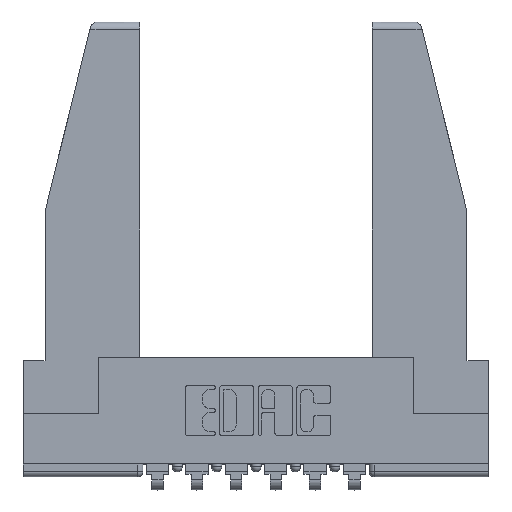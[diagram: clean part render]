
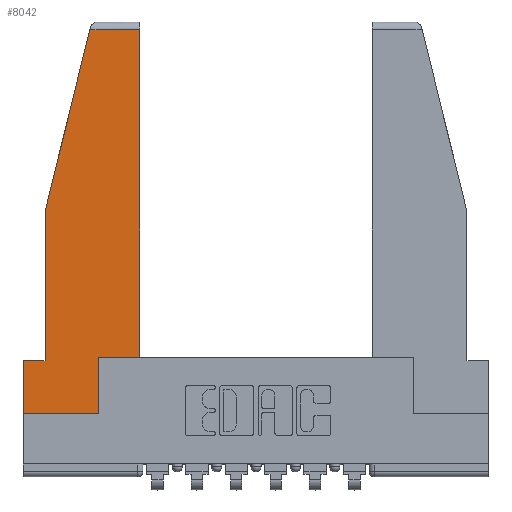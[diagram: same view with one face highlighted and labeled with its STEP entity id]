
A CAD part, top view. The second image highlights one B-rep face of the part: STEP entity #8042.
In plain terms, the highlighted planar face has unit normal (0, 0, 1).
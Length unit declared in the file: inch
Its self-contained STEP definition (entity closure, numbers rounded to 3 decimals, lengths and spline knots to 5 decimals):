
#149 = DIRECTION ( 'NONE',  ( 0., 1., 0. ) ) ;
#506 = EDGE_CURVE ( 'NONE', #4502, #9642, #3231, .T. ) ;
#559 = DIRECTION ( 'NONE',  ( -0.239, -0.971, 0. ) ) ;
#589 = VERTEX_POINT ( 'NONE', #7396 ) ;
#690 = CARTESIAN_POINT ( 'NONE',  ( 0.086, 0.8, 0. ) ) ;
#927 = CARTESIAN_POINT ( 'NONE',  ( 0.2636, 1.52, 0. ) ) ;
#933 = VECTOR ( 'NONE', #2830, 39.37008 ) ;
#1018 = CARTESIAN_POINT ( 'NONE',  ( 0.086, 0.21, 0. ) ) ;
#1309 = LINE ( 'NONE', #6070, #3878 ) ;
#1405 = EDGE_CURVE ( 'NONE', #5147, #3144, #2658, .T. ) ;
#1675 = FACE_OUTER_BOUND ( 'NONE', #10963, .T. ) ;
#1799 = CARTESIAN_POINT ( 'NONE',  ( 0., 0.21, 0. ) ) ;
#1808 = DIRECTION ( 'NONE',  ( 0., 0., 1. ) ) ;
#2299 = VECTOR ( 'NONE', #8438, 39.37008 ) ;
#2321 = DIRECTION ( 'NONE',  ( 1., 0., 0. ) ) ;
#2417 = CARTESIAN_POINT ( 'NONE',  ( 0.461, 0.223, 0. ) ) ;
#2658 = LINE ( 'NONE', #4690, #3226 ) ;
#2830 = DIRECTION ( 'NONE',  ( -1., 0., 0. ) ) ;
#2982 = ORIENTED_EDGE ( 'NONE', *, *, #9877, .T. ) ;
#3100 = VECTOR ( 'NONE', #149, 39.37008 ) ;
#3144 = VERTEX_POINT ( 'NONE', #12222 ) ;
#3226 = VECTOR ( 'NONE', #559, 39.37008 ) ;
#3231 = LINE ( 'NONE', #4208, #3100 ) ;
#3272 = EDGE_CURVE ( 'NONE', #589, #4502, #5633, .T. ) ;
#3565 = CARTESIAN_POINT ( 'NONE',  ( 0.297, 0., 0. ) ) ;
#3636 = PLANE ( 'NONE',  #4230 ) ;
#3766 = DIRECTION ( 'NONE',  ( 1., 0., 0. ) ) ;
#3878 = VECTOR ( 'NONE', #4056, 39.37008 ) ;
#4056 = DIRECTION ( 'NONE',  ( -1., 0., 0. ) ) ;
#4208 = CARTESIAN_POINT ( 'NONE',  ( 0.297, 0., 0. ) ) ;
#4230 = AXIS2_PLACEMENT_3D ( 'NONE', #12423, #1808, #3766 ) ;
#4235 = VERTEX_POINT ( 'NONE', #1018 ) ;
#4462 = EDGE_CURVE ( 'NONE', #9642, #12052, #11236, .T. ) ;
#4502 = VERTEX_POINT ( 'NONE', #3565 ) ;
#4690 = CARTESIAN_POINT ( 'NONE',  ( 0.271, 1.55, 0. ) ) ;
#4838 = ORIENTED_EDGE ( 'NONE', *, *, #4462, .T. ) ;
#5147 = VERTEX_POINT ( 'NONE', #927 ) ;
#5232 = VERTEX_POINT ( 'NONE', #11015 ) ;
#5301 = VECTOR ( 'NONE', #8489, 39.37008 ) ;
#5364 = CARTESIAN_POINT ( 'NONE',  ( 0.461, 0.223, 0. ) ) ;
#5633 = LINE ( 'NONE', #11498, #8528 ) ;
#5769 = EDGE_CURVE ( 'NONE', #3144, #4235, #9608, .T. ) ;
#6070 = CARTESIAN_POINT ( 'NONE',  ( 0., 1.52, 0. ) ) ;
#6345 = LINE ( 'NONE', #5364, #9210 ) ;
#7111 = ORIENTED_EDGE ( 'NONE', *, *, #8446, .T. ) ;
#7396 = CARTESIAN_POINT ( 'NONE',  ( 0., 0., 0. ) ) ;
#7596 = DIRECTION ( 'NONE',  ( 1., 0., 0. ) ) ;
#7936 = ORIENTED_EDGE ( 'NONE', *, *, #3272, .T. ) ;
#8042 = ADVANCED_FACE ( 'NONE', ( #1675 ), #3636, .T. ) ;
#8073 = VERTEX_POINT ( 'NONE', #9675 ) ;
#8438 = DIRECTION ( 'NONE',  ( 0., -1., 0. ) ) ;
#8446 = EDGE_CURVE ( 'NONE', #12052, #5232, #6345, .T. ) ;
#8489 = DIRECTION ( 'NONE',  ( 0., -1., 0. ) ) ;
#8528 = VECTOR ( 'NONE', #7596, 39.37008 ) ;
#9210 = VECTOR ( 'NONE', #9329, 39.37008 ) ;
#9329 = DIRECTION ( 'NONE',  ( 0., 1., 0. ) ) ;
#9608 = LINE ( 'NONE', #690, #2299 ) ;
#9642 = VERTEX_POINT ( 'NONE', #11294 ) ;
#9675 = CARTESIAN_POINT ( 'NONE',  ( 0., 0.21, 0. ) ) ;
#9854 = EDGE_CURVE ( 'NONE', #8073, #589, #10573, .T. ) ;
#9877 = EDGE_CURVE ( 'NONE', #4235, #8073, #10707, .T. ) ;
#10573 = LINE ( 'NONE', #12613, #5301 ) ;
#10707 = LINE ( 'NONE', #1799, #933 ) ;
#10788 = ORIENTED_EDGE ( 'NONE', *, *, #11911, .T. ) ;
#10963 = EDGE_LOOP ( 'NONE', ( #7111, #10788, #12024, #11926, #2982, #12049, #7936, #12226, #4838 ) ) ;
#11015 = CARTESIAN_POINT ( 'NONE',  ( 0.461, 1.52, 0. ) ) ;
#11236 = LINE ( 'NONE', #11367, #11433 ) ;
#11294 = CARTESIAN_POINT ( 'NONE',  ( 0.297, 0.223, 0. ) ) ;
#11367 = CARTESIAN_POINT ( 'NONE',  ( 0.297, 0.223, 0. ) ) ;
#11433 = VECTOR ( 'NONE', #2321, 39.37008 ) ;
#11498 = CARTESIAN_POINT ( 'NONE',  ( 0., 0., 0. ) ) ;
#11911 = EDGE_CURVE ( 'NONE', #5232, #5147, #1309, .T. ) ;
#11926 = ORIENTED_EDGE ( 'NONE', *, *, #5769, .T. ) ;
#12024 = ORIENTED_EDGE ( 'NONE', *, *, #1405, .T. ) ;
#12049 = ORIENTED_EDGE ( 'NONE', *, *, #9854, .T. ) ;
#12052 = VERTEX_POINT ( 'NONE', #2417 ) ;
#12222 = CARTESIAN_POINT ( 'NONE',  ( 0.086, 0.8, 0. ) ) ;
#12226 = ORIENTED_EDGE ( 'NONE', *, *, #506, .T. ) ;
#12423 = CARTESIAN_POINT ( 'NONE',  ( 0., 0., 0. ) ) ;
#12613 = CARTESIAN_POINT ( 'NONE',  ( 0., 0.21, 0. ) ) ;
